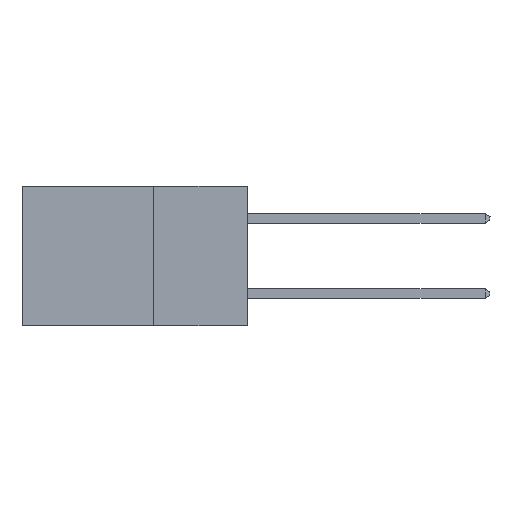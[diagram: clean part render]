
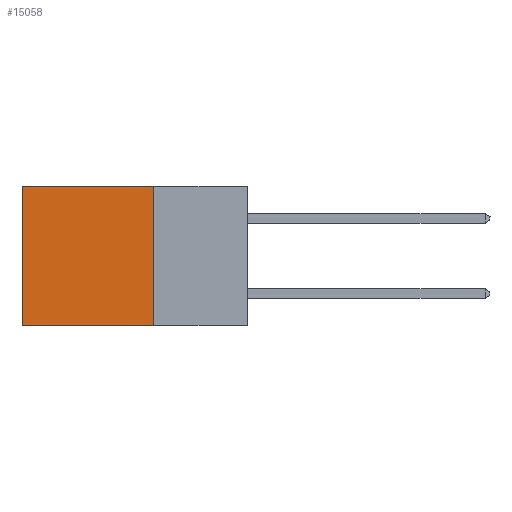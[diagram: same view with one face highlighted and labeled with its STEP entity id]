
A CAD part, left-side view. The second image highlights one B-rep face of the part: STEP entity #15058.
In plain terms, the highlighted planar face has unit normal (-1, 0, 0).
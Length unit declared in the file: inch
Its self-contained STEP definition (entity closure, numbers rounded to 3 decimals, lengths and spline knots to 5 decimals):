
#414 = EDGE_CURVE ( 'NONE', #15840, #14988, #21485, .T. ) ;
#3094 = CARTESIAN_POINT ( 'NONE',  ( 0.298, 0.25, 0. ) ) ;
#4325 = DIRECTION ( 'NONE',  ( 1., 0., 0. ) ) ;
#5079 = ORIENTED_EDGE ( 'NONE', *, *, #24705, .F. ) ;
#6606 = PLANE ( 'NONE',  #14634 ) ;
#8315 = DIRECTION ( 'NONE',  ( 0., 1., 0. ) ) ;
#8897 = VERTEX_POINT ( 'NONE', #11125 ) ;
#9186 = CARTESIAN_POINT ( 'NONE',  ( 0.298, 0.25, 0. ) ) ;
#10536 = CARTESIAN_POINT ( 'NONE',  ( 0.298, 0.6, 0. ) ) ;
#11125 = CARTESIAN_POINT ( 'NONE',  ( 0.298, 0.25, -0.37 ) ) ;
#12857 = DIRECTION ( 'NONE',  ( 0., 0., -1. ) ) ;
#13273 = EDGE_CURVE ( 'NONE', #14988, #27840, #14759, .T. ) ;
#14634 = AXIS2_PLACEMENT_3D ( 'NONE', #27376, #4325, #20594 ) ;
#14759 = LINE ( 'NONE', #10536, #25543 ) ;
#14988 = VERTEX_POINT ( 'NONE', #20299 ) ;
#15058 = ADVANCED_FACE ( 'NONE', ( #25121 ), #6606, .F. ) ;
#15840 = VERTEX_POINT ( 'NONE', #9186 ) ;
#17843 = ORIENTED_EDGE ( 'NONE', *, *, #13273, .T. ) ;
#18682 = CARTESIAN_POINT ( 'NONE',  ( 0.298, 0.6, -0.37 ) ) ;
#18776 = LINE ( 'NONE', #22192, #20240 ) ;
#19230 = CARTESIAN_POINT ( 'NONE',  ( 0.298, 0.25, 0. ) ) ;
#20240 = VECTOR ( 'NONE', #8315, 39.37008 ) ;
#20299 = CARTESIAN_POINT ( 'NONE',  ( 0.298, 0.6, 0. ) ) ;
#20594 = DIRECTION ( 'NONE',  ( 0., 0., -1. ) ) ;
#21485 = LINE ( 'NONE', #19230, #27535 ) ;
#21692 = DIRECTION ( 'NONE',  ( 0., 0., -1. ) ) ;
#22192 = CARTESIAN_POINT ( 'NONE',  ( 0.298, 0.25, -0.37 ) ) ;
#23314 = LINE ( 'NONE', #3094, #28664 ) ;
#24705 = EDGE_CURVE ( 'NONE', #8897, #27840, #18776, .T. ) ;
#25121 = FACE_OUTER_BOUND ( 'NONE', #25932, .T. ) ;
#25543 = VECTOR ( 'NONE', #12857, 39.37008 ) ;
#25910 = ORIENTED_EDGE ( 'NONE', *, *, #414, .T. ) ;
#25932 = EDGE_LOOP ( 'NONE', ( #17843, #5079, #28212, #25910 ) ) ;
#26504 = EDGE_CURVE ( 'NONE', #15840, #8897, #23314, .T. ) ;
#27376 = CARTESIAN_POINT ( 'NONE',  ( 0.298, 0.25, 0. ) ) ;
#27535 = VECTOR ( 'NONE', #27536, 39.37008 ) ;
#27536 = DIRECTION ( 'NONE',  ( 0., 1., 0. ) ) ;
#27840 = VERTEX_POINT ( 'NONE', #18682 ) ;
#28212 = ORIENTED_EDGE ( 'NONE', *, *, #26504, .F. ) ;
#28664 = VECTOR ( 'NONE', #21692, 39.37008 ) ;
